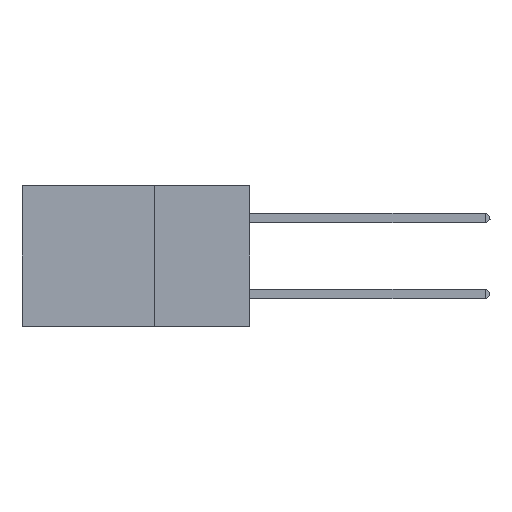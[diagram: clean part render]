
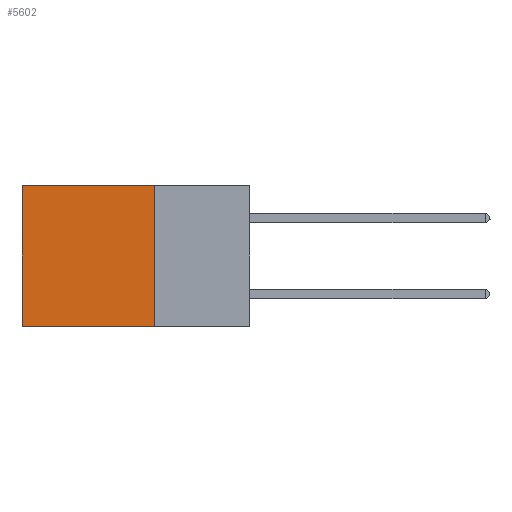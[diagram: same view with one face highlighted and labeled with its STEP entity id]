
A CAD part, left-side view. The second image highlights one B-rep face of the part: STEP entity #5602.
In plain terms, the highlighted planar face has unit normal (-1, 0, 0).
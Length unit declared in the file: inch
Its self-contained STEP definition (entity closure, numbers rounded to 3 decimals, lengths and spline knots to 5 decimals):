
#268 = DIRECTION ( 'NONE',  ( 0., 0., -1. ) ) ;
#361 = DIRECTION ( 'NONE',  ( 0., 0., -1. ) ) ;
#808 = CARTESIAN_POINT ( 'NONE',  ( 0.2875, 0.6, 0. ) ) ;
#1033 = CARTESIAN_POINT ( 'NONE',  ( 0.2875, 0.25, 0. ) ) ;
#1971 = CARTESIAN_POINT ( 'NONE',  ( 0.2875, 0.25, -0.37 ) ) ;
#2659 = VERTEX_POINT ( 'NONE', #1971 ) ;
#2819 = EDGE_CURVE ( 'NONE', #3193, #6873, #4917, .T. ) ;
#3193 = VERTEX_POINT ( 'NONE', #4567 ) ;
#3725 = FACE_OUTER_BOUND ( 'NONE', #5478, .T. ) ;
#4567 = CARTESIAN_POINT ( 'NONE',  ( 0.2875, 0.25, 0. ) ) ;
#4812 = CARTESIAN_POINT ( 'NONE',  ( 0.2875, 0.25, -0.37 ) ) ;
#4917 = LINE ( 'NONE', #5082, #11352 ) ;
#4942 = AXIS2_PLACEMENT_3D ( 'NONE', #1033, #5036, #16918 ) ;
#5036 = DIRECTION ( 'NONE',  ( 1., 0., 0. ) ) ;
#5082 = CARTESIAN_POINT ( 'NONE',  ( 0.2875, 0.25, 0. ) ) ;
#5478 = EDGE_LOOP ( 'NONE', ( #13665, #16515, #7046, #15974 ) ) ;
#5602 = ADVANCED_FACE ( 'NONE', ( #3725 ), #10159, .F. ) ;
#5953 = DIRECTION ( 'NONE',  ( 0., 1., 0. ) ) ;
#6505 = VECTOR ( 'NONE', #361, 39.37008 ) ;
#6702 = LINE ( 'NONE', #9305, #6505 ) ;
#6873 = VERTEX_POINT ( 'NONE', #808 ) ;
#7046 = ORIENTED_EDGE ( 'NONE', *, *, #11153, .F. ) ;
#7137 = EDGE_CURVE ( 'NONE', #6873, #10468, #16077, .T. ) ;
#8007 = EDGE_CURVE ( 'NONE', #2659, #10468, #12695, .T. ) ;
#8902 = DIRECTION ( 'NONE',  ( 0., 1., 0. ) ) ;
#9275 = VECTOR ( 'NONE', #5953, 39.37008 ) ;
#9305 = CARTESIAN_POINT ( 'NONE',  ( 0.2875, 0.25, 0. ) ) ;
#10159 = PLANE ( 'NONE',  #4942 ) ;
#10468 = VERTEX_POINT ( 'NONE', #11425 ) ;
#11153 = EDGE_CURVE ( 'NONE', #3193, #2659, #6702, .T. ) ;
#11352 = VECTOR ( 'NONE', #8902, 39.37008 ) ;
#11425 = CARTESIAN_POINT ( 'NONE',  ( 0.2875, 0.6, -0.37 ) ) ;
#12695 = LINE ( 'NONE', #4812, #9275 ) ;
#13665 = ORIENTED_EDGE ( 'NONE', *, *, #7137, .T. ) ;
#13675 = VECTOR ( 'NONE', #268, 39.37008 ) ;
#13876 = CARTESIAN_POINT ( 'NONE',  ( 0.2875, 0.6, 0. ) ) ;
#15974 = ORIENTED_EDGE ( 'NONE', *, *, #2819, .T. ) ;
#16077 = LINE ( 'NONE', #13876, #13675 ) ;
#16515 = ORIENTED_EDGE ( 'NONE', *, *, #8007, .F. ) ;
#16918 = DIRECTION ( 'NONE',  ( 0., 0., -1. ) ) ;
